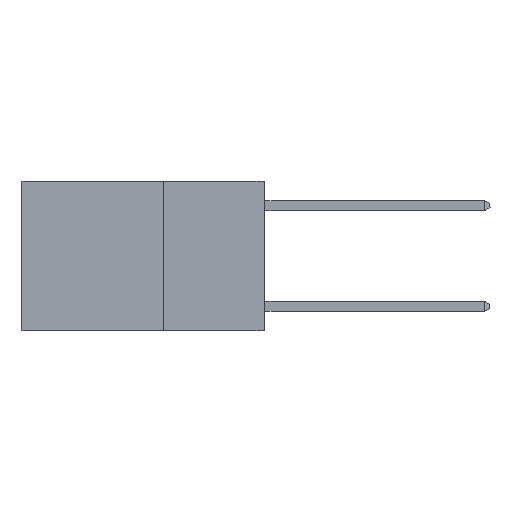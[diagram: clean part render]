
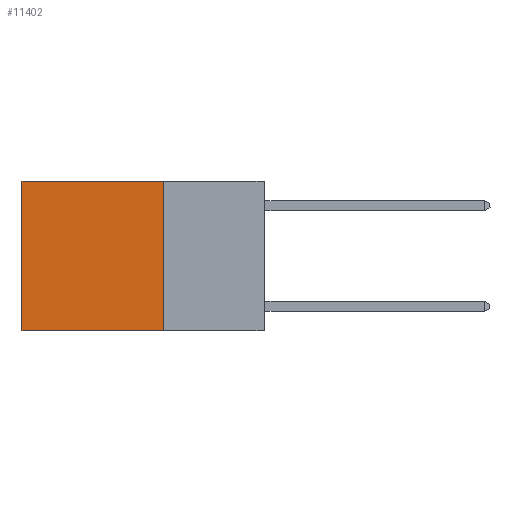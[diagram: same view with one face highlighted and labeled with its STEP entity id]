
A CAD part, left-side view. The second image highlights one B-rep face of the part: STEP entity #11402.
In plain terms, the highlighted planar face has unit normal (-1, 0, 0).
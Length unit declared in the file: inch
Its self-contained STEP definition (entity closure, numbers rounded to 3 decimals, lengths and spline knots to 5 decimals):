
#98 = DIRECTION ( 'NONE',  ( 1., 0., 0. ) ) ;
#517 = EDGE_CURVE ( 'NONE', #11216, #8875, #13653, .T. ) ;
#1066 = VECTOR ( 'NONE', #6930, 39.37008 ) ;
#1300 = CARTESIAN_POINT ( 'NONE',  ( 0.2625, 0.6, 0. ) ) ;
#1497 = CARTESIAN_POINT ( 'NONE',  ( 0.2625, 0.25, 0. ) ) ;
#1907 = EDGE_CURVE ( 'NONE', #6594, #7266, #7155, .T. ) ;
#2288 = AXIS2_PLACEMENT_3D ( 'NONE', #2393, #98, #6083 ) ;
#2393 = CARTESIAN_POINT ( 'NONE',  ( 0.2625, 0.25, 0. ) ) ;
#2410 = LINE ( 'NONE', #1497, #2754 ) ;
#2528 = ORIENTED_EDGE ( 'NONE', *, *, #517, .F. ) ;
#2671 = DIRECTION ( 'NONE',  ( 0., 1., 0. ) ) ;
#2754 = VECTOR ( 'NONE', #13472, 39.37008 ) ;
#2774 = FACE_OUTER_BOUND ( 'NONE', #3004, .T. ) ;
#3004 = EDGE_LOOP ( 'NONE', ( #7187, #7256, #2528, #4144 ) ) ;
#3864 = EDGE_CURVE ( 'NONE', #8875, #7266, #4346, .T. ) ;
#4144 = ORIENTED_EDGE ( 'NONE', *, *, #9142, .T. ) ;
#4346 = LINE ( 'NONE', #11186, #9317 ) ;
#4576 = CARTESIAN_POINT ( 'NONE',  ( 0.2625, 0.6, 0. ) ) ;
#4992 = DIRECTION ( 'NONE',  ( 0., 0., -1. ) ) ;
#6083 = DIRECTION ( 'NONE',  ( 0., 0., -1. ) ) ;
#6594 = VERTEX_POINT ( 'NONE', #4576 ) ;
#6887 = CARTESIAN_POINT ( 'NONE',  ( 0.2625, 0.25, -0.37 ) ) ;
#6930 = DIRECTION ( 'NONE',  ( 0., 0., -1. ) ) ;
#7155 = LINE ( 'NONE', #1300, #11888 ) ;
#7187 = ORIENTED_EDGE ( 'NONE', *, *, #1907, .T. ) ;
#7256 = ORIENTED_EDGE ( 'NONE', *, *, #3864, .F. ) ;
#7266 = VERTEX_POINT ( 'NONE', #10290 ) ;
#8758 = CARTESIAN_POINT ( 'NONE',  ( 0.2625, 0.25, 0. ) ) ;
#8875 = VERTEX_POINT ( 'NONE', #6887 ) ;
#9142 = EDGE_CURVE ( 'NONE', #11216, #6594, #2410, .T. ) ;
#9317 = VECTOR ( 'NONE', #2671, 39.37008 ) ;
#10290 = CARTESIAN_POINT ( 'NONE',  ( 0.2625, 0.6, -0.37 ) ) ;
#10887 = CARTESIAN_POINT ( 'NONE',  ( 0.2625, 0.25, 0. ) ) ;
#11186 = CARTESIAN_POINT ( 'NONE',  ( 0.2625, 0.25, -0.37 ) ) ;
#11216 = VERTEX_POINT ( 'NONE', #10887 ) ;
#11402 = ADVANCED_FACE ( 'NONE', ( #2774 ), #11946, .F. ) ;
#11888 = VECTOR ( 'NONE', #4992, 39.37008 ) ;
#11946 = PLANE ( 'NONE',  #2288 ) ;
#13472 = DIRECTION ( 'NONE',  ( 0., 1., 0. ) ) ;
#13653 = LINE ( 'NONE', #8758, #1066 ) ;
